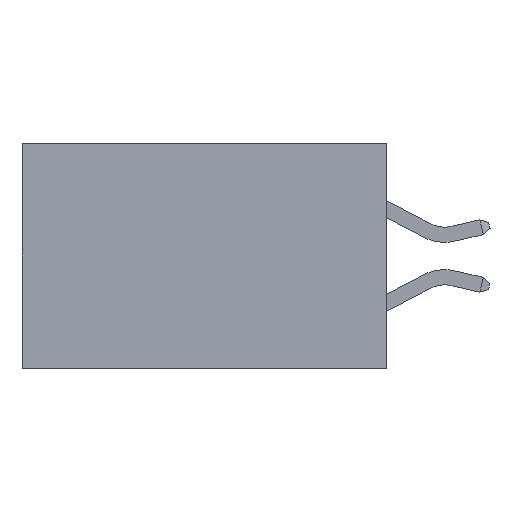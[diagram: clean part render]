
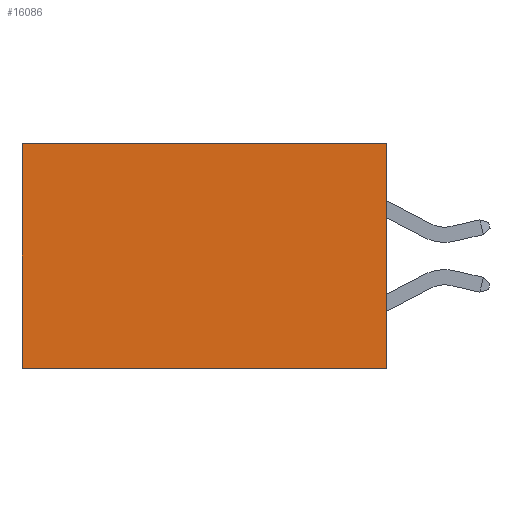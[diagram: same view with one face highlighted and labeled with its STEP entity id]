
A CAD part, left-side view. The second image highlights one B-rep face of the part: STEP entity #16086.
In plain terms, the highlighted planar face has unit normal (-1, 0, 0).
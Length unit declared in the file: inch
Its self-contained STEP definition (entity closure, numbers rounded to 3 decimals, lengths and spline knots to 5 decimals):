
#52 = FACE_OUTER_BOUND ( 'NONE', #18327, .T. ) ;
#461 = VERTEX_POINT ( 'NONE', #18687 ) ;
#468 = CARTESIAN_POINT ( 'NONE',  ( 0.298, 0.6, -0.37 ) ) ;
#1297 = CARTESIAN_POINT ( 'NONE',  ( 0.298, 0., 0. ) ) ;
#5067 = CARTESIAN_POINT ( 'NONE',  ( 0.298, 0., 0. ) ) ;
#6114 = CARTESIAN_POINT ( 'NONE',  ( 0.298, 0., 0. ) ) ;
#7419 = DIRECTION ( 'NONE',  ( 0., 1., 0. ) ) ;
#8182 = VERTEX_POINT ( 'NONE', #27714 ) ;
#8290 = AXIS2_PLACEMENT_3D ( 'NONE', #1297, #8302, #24494 ) ;
#8302 = DIRECTION ( 'NONE',  ( 1., 0., 0. ) ) ;
#8422 = DIRECTION ( 'NONE',  ( 0., 1., 0. ) ) ;
#8522 = CARTESIAN_POINT ( 'NONE',  ( 0.298, 0., -0.37 ) ) ;
#8674 = DIRECTION ( 'NONE',  ( 0., 0., -1. ) ) ;
#10298 = VERTEX_POINT ( 'NONE', #19533 ) ;
#10795 = DIRECTION ( 'NONE',  ( 0., 0., -1. ) ) ;
#11614 = LINE ( 'NONE', #20234, #22479 ) ;
#14122 = LINE ( 'NONE', #8522, #19525 ) ;
#14309 = ORIENTED_EDGE ( 'NONE', *, *, #15421, .F. ) ;
#14745 = ORIENTED_EDGE ( 'NONE', *, *, #28985, .T. ) ;
#15421 = EDGE_CURVE ( 'NONE', #8182, #461, #23671, .T. ) ;
#16086 = ADVANCED_FACE ( 'NONE', ( #52 ), #22189, .F. ) ;
#16791 = EDGE_CURVE ( 'NONE', #10298, #23871, #11614, .T. ) ;
#18327 = EDGE_LOOP ( 'NONE', ( #18420, #24318, #14309, #14745 ) ) ;
#18420 = ORIENTED_EDGE ( 'NONE', *, *, #16791, .T. ) ;
#18687 = CARTESIAN_POINT ( 'NONE',  ( 0.298, 0., -0.37 ) ) ;
#19321 = VECTOR ( 'NONE', #7419, 39.37008 ) ;
#19525 = VECTOR ( 'NONE', #8422, 39.37008 ) ;
#19533 = CARTESIAN_POINT ( 'NONE',  ( 0.298, 0.6, 0. ) ) ;
#20234 = CARTESIAN_POINT ( 'NONE',  ( 0.298, 0.6, 0. ) ) ;
#20713 = EDGE_CURVE ( 'NONE', #461, #23871, #14122, .T. ) ;
#22189 = PLANE ( 'NONE',  #8290 ) ;
#22479 = VECTOR ( 'NONE', #8674, 39.37008 ) ;
#22939 = VECTOR ( 'NONE', #10795, 39.37008 ) ;
#23671 = LINE ( 'NONE', #6114, #22939 ) ;
#23871 = VERTEX_POINT ( 'NONE', #468 ) ;
#24318 = ORIENTED_EDGE ( 'NONE', *, *, #20713, .F. ) ;
#24494 = DIRECTION ( 'NONE',  ( 0., 0., -1. ) ) ;
#26153 = LINE ( 'NONE', #5067, #19321 ) ;
#27714 = CARTESIAN_POINT ( 'NONE',  ( 0.298, 0., 0. ) ) ;
#28985 = EDGE_CURVE ( 'NONE', #8182, #10298, #26153, .T. ) ;
